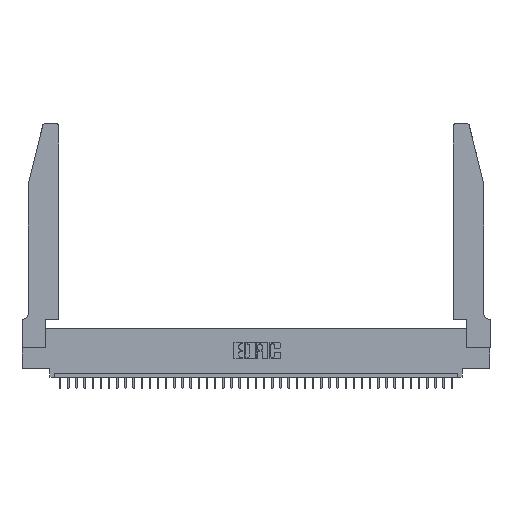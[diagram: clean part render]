
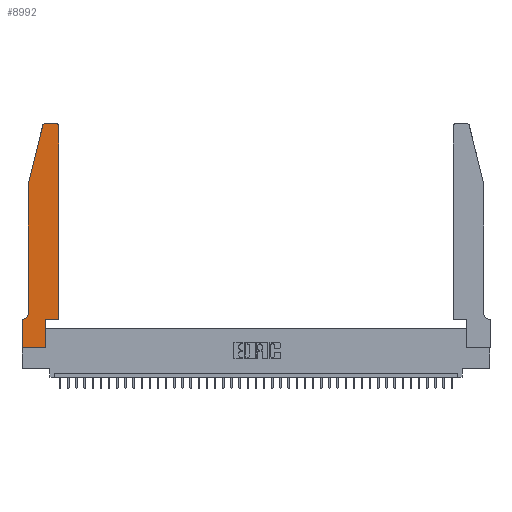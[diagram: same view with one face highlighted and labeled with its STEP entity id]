
A CAD part, top view. The second image highlights one B-rep face of the part: STEP entity #8992.
In plain terms, the highlighted planar face has unit normal (0, 0, 1).
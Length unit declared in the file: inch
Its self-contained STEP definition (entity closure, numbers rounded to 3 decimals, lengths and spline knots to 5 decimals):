
#458 = EDGE_CURVE ( 'NONE', #8606, #9414, #29755, .T. ) ;
#1241 = CARTESIAN_POINT ( 'NONE',  ( 0.0055, 0.42, 0.37 ) ) ;
#1542 = AXIS2_PLACEMENT_3D ( 'NONE', #1241, #20908, #32706 ) ;
#1785 = ORIENTED_EDGE ( 'NONE', *, *, #27511, .T. ) ;
#2672 = ORIENTED_EDGE ( 'NONE', *, *, #38111, .T. ) ;
#2883 = ORIENTED_EDGE ( 'NONE', *, *, #5278, .T. ) ;
#3108 = CARTESIAN_POINT ( 'NONE',  ( 0.4505, 0.35, 0.37 ) ) ;
#4225 = EDGE_CURVE ( 'NONE', #15540, #13161, #35333, .T. ) ;
#5032 = VERTEX_POINT ( 'NONE', #8882 ) ;
#5044 = CARTESIAN_POINT ( 'NONE',  ( 0.0755, 2., 0.37 ) ) ;
#5278 = EDGE_CURVE ( 'NONE', #18381, #8606, #37576, .T. ) ;
#5373 = VECTOR ( 'NONE', #24560, 39.37008 ) ;
#7288 = ORIENTED_EDGE ( 'NONE', *, *, #27051, .T. ) ;
#7291 = DIRECTION ( 'NONE',  ( 0., -1., 0. ) ) ;
#7343 = CARTESIAN_POINT ( 'NONE',  ( 0.4505, 0.35, 0.37 ) ) ;
#7747 = DIRECTION ( 'NONE',  ( 1., 0., 0. ) ) ;
#8606 = VERTEX_POINT ( 'NONE', #21421 ) ;
#8882 = CARTESIAN_POINT ( 'NONE',  ( 0.0755, 0.42, 0.37 ) ) ;
#8992 = ADVANCED_FACE ( 'NONE', ( #35463 ), #28839, .T. ) ;
#9403 = VECTOR ( 'NONE', #16662, 39.37008 ) ;
#9414 = VERTEX_POINT ( 'NONE', #3108 ) ;
#10362 = LINE ( 'NONE', #23025, #17071 ) ;
#10506 = CARTESIAN_POINT ( 'NONE',  ( 0.284, 2.72, 0.37 ) ) ;
#10613 = CARTESIAN_POINT ( 'NONE',  ( 0.0055, 0.35, 0.37 ) ) ;
#10712 = DIRECTION ( 'NONE',  ( 1., 0., 0. ) ) ;
#12141 = CARTESIAN_POINT ( 'NONE',  ( 0.25487, 2.72718, 0.37 ) ) ;
#12430 = ORIENTED_EDGE ( 'NONE', *, *, #26165, .T. ) ;
#12514 = CARTESIAN_POINT ( 'NONE',  ( 0.0755, 2., 0.37 ) ) ;
#13161 = VERTEX_POINT ( 'NONE', #36641 ) ;
#13274 = DIRECTION ( 'NONE',  ( -1., 0., 0. ) ) ;
#13531 = DIRECTION ( 'NONE',  ( 0., 0., 1. ) ) ;
#14649 = VECTOR ( 'NONE', #32411, 39.37008 ) ;
#15239 = CARTESIAN_POINT ( 'NONE',  ( 0.2865, 0.35, 0.37 ) ) ;
#15335 = EDGE_CURVE ( 'NONE', #9414, #30893, #17262, .T. ) ;
#15540 = VERTEX_POINT ( 'NONE', #31715 ) ;
#15981 = AXIS2_PLACEMENT_3D ( 'NONE', #10506, #28758, #23165 ) ;
#16662 = DIRECTION ( 'NONE',  ( 0., 1., 0. ) ) ;
#16694 = CARTESIAN_POINT ( 'NONE',  ( 0., 0., 0.37 ) ) ;
#16848 = CARTESIAN_POINT ( 'NONE',  ( 0.4205, 2.72, 0.37 ) ) ;
#17071 = VECTOR ( 'NONE', #7291, 39.37008 ) ;
#17240 = VECTOR ( 'NONE', #31746, 39.37008 ) ;
#17262 = LINE ( 'NONE', #7343, #9403 ) ;
#18102 = EDGE_CURVE ( 'NONE', #5032, #27525, #19409, .T. ) ;
#18381 = VERTEX_POINT ( 'NONE', #32053 ) ;
#19292 = CARTESIAN_POINT ( 'NONE',  ( 0.0755, 0.35, 0.37 ) ) ;
#19409 = CIRCLE ( 'NONE', #1542, 0.07 ) ;
#19666 = VECTOR ( 'NONE', #38578, 39.37008 ) ;
#20379 = ORIENTED_EDGE ( 'NONE', *, *, #27553, .T. ) ;
#20385 = AXIS2_PLACEMENT_3D ( 'NONE', #25764, #25554, #38349 ) ;
#20908 = DIRECTION ( 'NONE',  ( 0., 0., -1. ) ) ;
#21421 = CARTESIAN_POINT ( 'NONE',  ( 0.2865, 0.35, 0.37 ) ) ;
#21859 = ORIENTED_EDGE ( 'NONE', *, *, #39361, .T. ) ;
#21971 = AXIS2_PLACEMENT_3D ( 'NONE', #16848, #13531, #7747 ) ;
#22437 = ORIENTED_EDGE ( 'NONE', *, *, #18102, .T. ) ;
#22493 = EDGE_LOOP ( 'NONE', ( #12430, #7288, #21859, #2672, #22437, #27930, #32126, #1785, #2883, #26802, #34795, #20379 ) ) ;
#22601 = CIRCLE ( 'NONE', #15981, 0.03 ) ;
#22906 = CARTESIAN_POINT ( 'NONE',  ( 0.4505, 2.72, 0.37 ) ) ;
#23025 = CARTESIAN_POINT ( 'NONE',  ( 0.0755, 2., 0.37 ) ) ;
#23165 = DIRECTION ( 'NONE',  ( 1., 0., 0. ) ) ;
#23561 = CARTESIAN_POINT ( 'NONE',  ( 0.4505, 0.35, 0.37 ) ) ;
#23678 = DIRECTION ( 'NONE',  ( 1., 0., 0. ) ) ;
#24560 = DIRECTION ( 'NONE',  ( 0., 1., 0. ) ) ;
#24667 = VERTEX_POINT ( 'NONE', #25903 ) ;
#25362 = CARTESIAN_POINT ( 'NONE',  ( 0.2605, 2.75, 0.37 ) ) ;
#25554 = DIRECTION ( 'NONE',  ( 0., 0., 1. ) ) ;
#25764 = CARTESIAN_POINT ( 'NONE',  ( 0., 0.35, 0.37 ) ) ;
#25903 = CARTESIAN_POINT ( 'NONE',  ( 0.284, 2.75, 0.37 ) ) ;
#26165 = EDGE_CURVE ( 'NONE', #27655, #24667, #38360, .T. ) ;
#26366 = LINE ( 'NONE', #32761, #36475 ) ;
#26802 = ORIENTED_EDGE ( 'NONE', *, *, #458, .T. ) ;
#27051 = EDGE_CURVE ( 'NONE', #24667, #37532, #22601, .T. ) ;
#27511 = EDGE_CURVE ( 'NONE', #13161, #18381, #26366, .T. ) ;
#27525 = VERTEX_POINT ( 'NONE', #10613 ) ;
#27553 = EDGE_CURVE ( 'NONE', #30893, #27655, #39780, .T. ) ;
#27655 = VERTEX_POINT ( 'NONE', #40003 ) ;
#27930 = ORIENTED_EDGE ( 'NONE', *, *, #35093, .T. ) ;
#28758 = DIRECTION ( 'NONE',  ( 0., 0., 1. ) ) ;
#28839 = PLANE ( 'NONE',  #20385 ) ;
#29755 = LINE ( 'NONE', #23561, #36332 ) ;
#30271 = VERTEX_POINT ( 'NONE', #5044 ) ;
#30893 = VERTEX_POINT ( 'NONE', #22906 ) ;
#31551 = LINE ( 'NONE', #12514, #19666 ) ;
#31715 = CARTESIAN_POINT ( 'NONE',  ( 0., 0.35, 0.37 ) ) ;
#31746 = DIRECTION ( 'NONE',  ( -1., 0., 0. ) ) ;
#32053 = CARTESIAN_POINT ( 'NONE',  ( 0.2865, 0., 0.37 ) ) ;
#32126 = ORIENTED_EDGE ( 'NONE', *, *, #4225, .T. ) ;
#32411 = DIRECTION ( 'NONE',  ( 0., -1., 0. ) ) ;
#32706 = DIRECTION ( 'NONE',  ( -1., 0., 0. ) ) ;
#32761 = CARTESIAN_POINT ( 'NONE',  ( 0., 0., 0.37 ) ) ;
#33406 = VECTOR ( 'NONE', #13274, 39.37008 ) ;
#34795 = ORIENTED_EDGE ( 'NONE', *, *, #15335, .T. ) ;
#35093 = EDGE_CURVE ( 'NONE', #27525, #15540, #37901, .T. ) ;
#35333 = LINE ( 'NONE', #16694, #14649 ) ;
#35463 = FACE_OUTER_BOUND ( 'NONE', #22493, .T. ) ;
#36332 = VECTOR ( 'NONE', #10712, 39.37008 ) ;
#36475 = VECTOR ( 'NONE', #23678, 39.37008 ) ;
#36641 = CARTESIAN_POINT ( 'NONE',  ( 0., 0., 0.37 ) ) ;
#37532 = VERTEX_POINT ( 'NONE', #12141 ) ;
#37576 = LINE ( 'NONE', #15239, #5373 ) ;
#37901 = LINE ( 'NONE', #19292, #33406 ) ;
#38111 = EDGE_CURVE ( 'NONE', #30271, #5032, #10362, .T. ) ;
#38349 = DIRECTION ( 'NONE',  ( 1., 0., 0. ) ) ;
#38360 = LINE ( 'NONE', #25362, #17240 ) ;
#38578 = DIRECTION ( 'NONE',  ( -0.239, -0.971, 0. ) ) ;
#39361 = EDGE_CURVE ( 'NONE', #37532, #30271, #31551, .T. ) ;
#39780 = CIRCLE ( 'NONE', #21971, 0.03 ) ;
#40003 = CARTESIAN_POINT ( 'NONE',  ( 0.4205, 2.75, 0.37 ) ) ;
